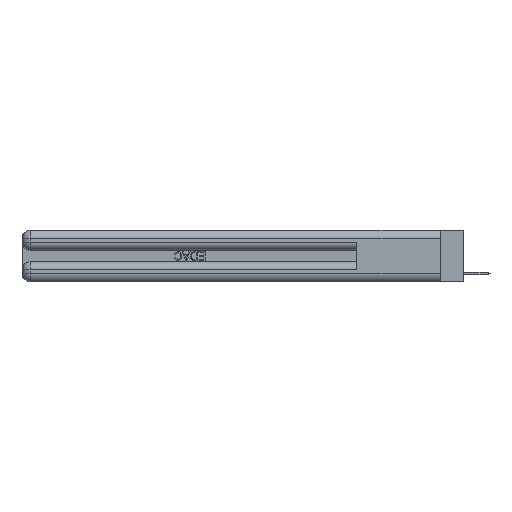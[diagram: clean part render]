
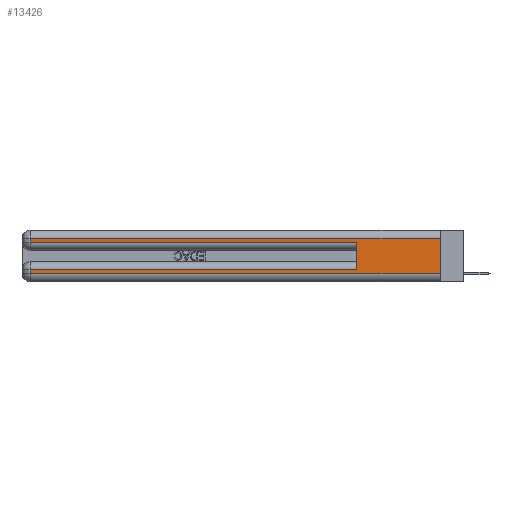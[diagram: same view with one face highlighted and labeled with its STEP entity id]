
A CAD part, left-side view. The second image highlights one B-rep face of the part: STEP entity #13426.
In plain terms, the highlighted planar face has unit normal (-1, 0, 0).
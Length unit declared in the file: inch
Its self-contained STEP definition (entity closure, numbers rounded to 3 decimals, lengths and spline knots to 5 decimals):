
#1241 = EDGE_CURVE ( 'NONE', #24671, #7549, #20036, .T. ) ;
#1326 = ORIENTED_EDGE ( 'NONE', *, *, #2269, .T. ) ;
#2262 = CARTESIAN_POINT ( 'NONE',  ( 0., 0., 0.06 ) ) ;
#2269 = EDGE_CURVE ( 'NONE', #5302, #11312, #12127, .T. ) ;
#2389 = DIRECTION ( 'NONE',  ( 1., 0., 0. ) ) ;
#2419 = DIRECTION ( 'NONE',  ( 0., 0., 1. ) ) ;
#3319 = DIRECTION ( 'NONE',  ( 0., 1., 0. ) ) ;
#3555 = LINE ( 'NONE', #24069, #17813 ) ;
#4169 = DIRECTION ( 'NONE',  ( 0., 0., -1. ) ) ;
#4437 = VERTEX_POINT ( 'NONE', #12132 ) ;
#5302 = VERTEX_POINT ( 'NONE', #20386 ) ;
#5401 = ORIENTED_EDGE ( 'NONE', *, *, #1241, .T. ) ;
#5432 = LINE ( 'NONE', #21888, #30360 ) ;
#5728 = FACE_OUTER_BOUND ( 'NONE', #33607, .T. ) ;
#6254 = EDGE_CURVE ( 'NONE', #24671, #15176, #6367, .T. ) ;
#6367 = LINE ( 'NONE', #33107, #18942 ) ;
#6397 = AXIS2_PLACEMENT_3D ( 'NONE', #31947, #2389, #8304 ) ;
#7549 = VERTEX_POINT ( 'NONE', #13061 ) ;
#7857 = VECTOR ( 'NONE', #16335, 39.37008 ) ;
#8304 = DIRECTION ( 'NONE',  ( 0., 0., -1. ) ) ;
#9664 = ORIENTED_EDGE ( 'NONE', *, *, #6254, .F. ) ;
#9894 = CARTESIAN_POINT ( 'NONE',  ( 0., 0., 0.31 ) ) ;
#10259 = EDGE_CURVE ( 'NONE', #7549, #29683, #11808, .T. ) ;
#10517 = ORIENTED_EDGE ( 'NONE', *, *, #26476, .F. ) ;
#10596 = CARTESIAN_POINT ( 'NONE',  ( 0., 0., 0.06 ) ) ;
#11312 = VERTEX_POINT ( 'NONE', #28068 ) ;
#11361 = DIRECTION ( 'NONE',  ( 0., -1., 0. ) ) ;
#11808 = LINE ( 'NONE', #19797, #7857 ) ;
#11864 = VECTOR ( 'NONE', #2419, 39.37008 ) ;
#11973 = VECTOR ( 'NONE', #4169, 39.37008 ) ;
#12127 = LINE ( 'NONE', #28002, #11973 ) ;
#12132 = CARTESIAN_POINT ( 'NONE',  ( 0., 0.6, 0.085 ) ) ;
#12220 = CARTESIAN_POINT ( 'NONE',  ( 0., 0., 0.31 ) ) ;
#13061 = CARTESIAN_POINT ( 'NONE',  ( 0., 2.94, 0.31 ) ) ;
#13375 = VERTEX_POINT ( 'NONE', #33351 ) ;
#13426 = ADVANCED_FACE ( 'NONE', ( #5728 ), #28996, .F. ) ;
#14296 = DIRECTION ( 'NONE',  ( 0., 0., -1. ) ) ;
#15176 = VERTEX_POINT ( 'NONE', #2262 ) ;
#15329 = EDGE_CURVE ( 'NONE', #11312, #15176, #18421, .T. ) ;
#16335 = DIRECTION ( 'NONE',  ( 0., 0., -1. ) ) ;
#17813 = VECTOR ( 'NONE', #11361, 39.37008 ) ;
#17978 = CARTESIAN_POINT ( 'NONE',  ( 0., 2.94, 0.285 ) ) ;
#18421 = LINE ( 'NONE', #10596, #22105 ) ;
#18662 = EDGE_CURVE ( 'NONE', #29683, #13375, #3555, .T. ) ;
#18942 = VECTOR ( 'NONE', #14296, 39.37008 ) ;
#19797 = CARTESIAN_POINT ( 'NONE',  ( 0., 2.94, 0.37 ) ) ;
#20036 = LINE ( 'NONE', #12220, #22453 ) ;
#20386 = CARTESIAN_POINT ( 'NONE',  ( 0., 2.94, 0.085 ) ) ;
#21729 = EDGE_CURVE ( 'NONE', #4437, #5302, #5432, .T. ) ;
#21888 = CARTESIAN_POINT ( 'NONE',  ( 0., 0., 0.085 ) ) ;
#22105 = VECTOR ( 'NONE', #31833, 39.37008 ) ;
#22360 = ORIENTED_EDGE ( 'NONE', *, *, #10259, .T. ) ;
#22453 = VECTOR ( 'NONE', #30517, 39.37008 ) ;
#23064 = ORIENTED_EDGE ( 'NONE', *, *, #15329, .T. ) ;
#23448 = CARTESIAN_POINT ( 'NONE',  ( 0., 0.6, 0.145 ) ) ;
#24069 = CARTESIAN_POINT ( 'NONE',  ( 0., 0., 0.285 ) ) ;
#24671 = VERTEX_POINT ( 'NONE', #9894 ) ;
#25722 = LINE ( 'NONE', #23448, #11864 ) ;
#25896 = ORIENTED_EDGE ( 'NONE', *, *, #18662, .T. ) ;
#26476 = EDGE_CURVE ( 'NONE', #4437, #13375, #25722, .T. ) ;
#28002 = CARTESIAN_POINT ( 'NONE',  ( 0., 2.94, 0.37 ) ) ;
#28068 = CARTESIAN_POINT ( 'NONE',  ( 0., 2.94, 0.06 ) ) ;
#28996 = PLANE ( 'NONE',  #6397 ) ;
#29683 = VERTEX_POINT ( 'NONE', #17978 ) ;
#29968 = ORIENTED_EDGE ( 'NONE', *, *, #21729, .T. ) ;
#30360 = VECTOR ( 'NONE', #3319, 39.37008 ) ;
#30517 = DIRECTION ( 'NONE',  ( 0., 1., 0. ) ) ;
#31833 = DIRECTION ( 'NONE',  ( 0., -1., 0. ) ) ;
#31947 = CARTESIAN_POINT ( 'NONE',  ( 0., 0., 0.37 ) ) ;
#33107 = CARTESIAN_POINT ( 'NONE',  ( 0., 0., 0.37 ) ) ;
#33351 = CARTESIAN_POINT ( 'NONE',  ( 0., 0.6, 0.285 ) ) ;
#33607 = EDGE_LOOP ( 'NONE', ( #9664, #5401, #22360, #25896, #10517, #29968, #1326, #23064 ) ) ;
